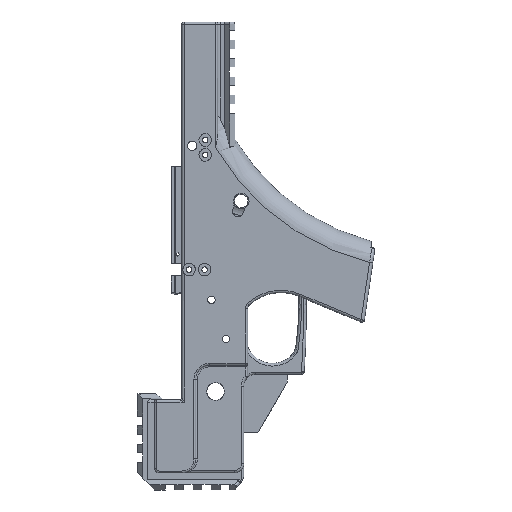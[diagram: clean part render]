
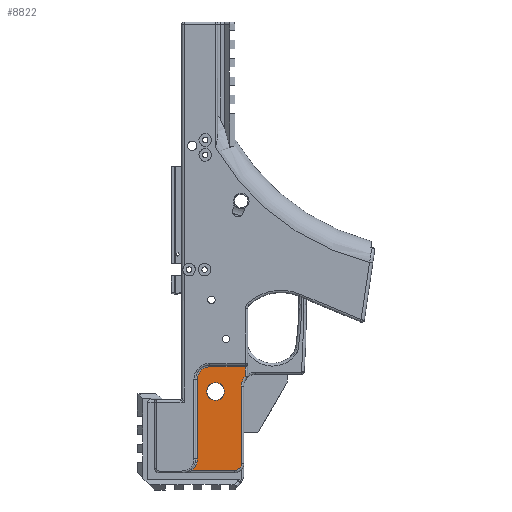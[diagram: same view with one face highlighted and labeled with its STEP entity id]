
A CAD part, left-side view. The second image highlights one B-rep face of the part: STEP entity #8822.
In plain terms, the highlighted planar face has unit normal (-1, 0, 0).
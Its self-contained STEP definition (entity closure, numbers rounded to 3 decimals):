
#103=FACE_BOUND('',#3094,.T.);
#339=CIRCLE('',#9271,7.62);
#341=CIRCLE('',#9275,3.81);
#360=CIRCLE('',#9303,6.752);
#365=CIRCLE('',#9311,8.488);
#433=CIRCLE('',#9473,4.826);
#786=LINE('',#13499,#1555);
#789=LINE('',#13516,#1558);
#793=LINE('',#13556,#1562);
#795=LINE('',#13569,#1564);
#995=LINE('',#14787,#1764);
#1555=VECTOR('',#10351,10.);
#1558=VECTOR('',#10366,10.);
#1562=VECTOR('',#10410,10.);
#1564=VECTOR('',#10426,10.);
#1764=VECTOR('',#10960,10.);
#2292=PLANE('',#9472);
#2583=FACE_OUTER_BOUND('',#3093,.T.);
#3093=EDGE_LOOP('',(#6664,#6665,#6666,#6667,#6668,#6669,#6670,#6671,#6672));
#3094=EDGE_LOOP('',(#6673));
#3860=VERTEX_POINT('',#13490);
#3862=VERTEX_POINT('',#13494);
#3863=VERTEX_POINT('',#13498);
#3865=VERTEX_POINT('',#13504);
#3867=VERTEX_POINT('',#13510);
#3882=VERTEX_POINT('',#13553);
#3883=VERTEX_POINT('',#13555);
#3885=VERTEX_POINT('',#13561);
#3887=VERTEX_POINT('',#13567);
#4108=VERTEX_POINT('',#14788);
#4751=EDGE_CURVE('',#3862,#3860,#339,.T.);
#4752=EDGE_CURVE('',#3860,#3863,#786,.T.);
#4755=EDGE_CURVE('',#3863,#3865,#341,.T.);
#4760=EDGE_CURVE('',#3865,#3867,#789,.T.);
#4777=EDGE_CURVE('',#3882,#3883,#793,.T.);
#4781=EDGE_CURVE('',#3885,#3882,#360,.T.);
#4784=EDGE_CURVE('',#3887,#3885,#795,.T.);
#4790=EDGE_CURVE('',#3867,#3887,#365,.T.);
#5099=EDGE_CURVE('',#3883,#3862,#995,.T.);
#5100=EDGE_CURVE('',#4108,#4108,#433,.T.);
#6664=ORIENTED_EDGE('',*,*,#4751,.F.);
#6665=ORIENTED_EDGE('',*,*,#5099,.F.);
#6666=ORIENTED_EDGE('',*,*,#4777,.F.);
#6667=ORIENTED_EDGE('',*,*,#4781,.F.);
#6668=ORIENTED_EDGE('',*,*,#4784,.F.);
#6669=ORIENTED_EDGE('',*,*,#4790,.F.);
#6670=ORIENTED_EDGE('',*,*,#4760,.F.);
#6671=ORIENTED_EDGE('',*,*,#4755,.F.);
#6672=ORIENTED_EDGE('',*,*,#4752,.F.);
#6673=ORIENTED_EDGE('',*,*,#5100,.T.);
#8822=ADVANCED_FACE('',(#2583,#103),#2292,.F.);
#9271=AXIS2_PLACEMENT_3D('',#13496,#10347,#10348);
#9275=AXIS2_PLACEMENT_3D('',#13505,#10357,#10358);
#9303=AXIS2_PLACEMENT_3D('',#13563,#10419,#10420);
#9311=AXIS2_PLACEMENT_3D('',#13602,#10438,#10439);
#9472=AXIS2_PLACEMENT_3D('',#14786,#10958,#10959);
#9473=AXIS2_PLACEMENT_3D('',#14789,#10961,#10962);
#10347=DIRECTION('center_axis',(-1.,0.,0.));
#10348=DIRECTION('ref_axis',(0.,0.928,0.373));
#10351=DIRECTION('',(0.,0.,-1.));
#10357=DIRECTION('center_axis',(1.,0.,0.));
#10358=DIRECTION('ref_axis',(0.,-0.707,-0.707));
#10366=DIRECTION('',(0.,1.,0.));
#10410=DIRECTION('',(0.,-1.,0.));
#10419=DIRECTION('center_axis',(1.,0.,0.));
#10420=DIRECTION('ref_axis',(0.,1.,0.));
#10426=DIRECTION('',(0.,0.,1.));
#10438=DIRECTION('center_axis',(-1.,0.,0.));
#10439=DIRECTION('ref_axis',(0.,-0.664,-0.748));
#10958=DIRECTION('center_axis',(1.,0.,0.));
#10959=DIRECTION('ref_axis',(0.,0.,-1.));
#10960=DIRECTION('',(0.,0.,-1.));
#10961=DIRECTION('center_axis',(1.,0.,0.));
#10962=DIRECTION('ref_axis',(0.,0.,-1.));
#13490=CARTESIAN_POINT('',(-11.43,-26.9,-130.907));
#13494=CARTESIAN_POINT('',(-11.43,-29.017,-125.636));
#13496=CARTESIAN_POINT('Origin',(-11.43,-34.52,-130.907));
#13498=CARTESIAN_POINT('',(-11.43,-26.9,-173.176));
#13499=CARTESIAN_POINT('',(-11.43,-26.9,-148.565));
#13504=CARTESIAN_POINT('',(-11.43,-23.09,-176.986));
#13505=CARTESIAN_POINT('Origin',(-11.43,-23.09,-173.176));
#13510=CARTESIAN_POINT('',(-11.43,-0.019,-176.986));
#13516=CARTESIAN_POINT('',(-11.43,-7.511,-176.986));
#13553=CARTESIAN_POINT('',(-11.43,-9.627,-120.454));
#13555=CARTESIAN_POINT('',(-11.43,-29.017,-120.454));
#13556=CARTESIAN_POINT('',(-11.43,-35.059,-120.454));
#13561=CARTESIAN_POINT('',(-11.43,-2.874,-127.206));
#13563=CARTESIAN_POINT('Origin',(-11.43,-9.627,-127.206));
#13567=CARTESIAN_POINT('',(-11.43,-2.874,-170.636));
#13569=CARTESIAN_POINT('',(-11.43,-2.874,-87.49));
#13602=CARTESIAN_POINT('Origin',(-11.43,5.613,-170.636));
#14786=CARTESIAN_POINT('Origin',(-11.43,-16.801,-129.514));
#14787=CARTESIAN_POINT('',(-11.43,-29.017,-161.99));
#14788=CARTESIAN_POINT('',(-11.43,-12.829,-129.103));
#14789=CARTESIAN_POINT('Origin',(-11.43,-12.829,-133.929));
